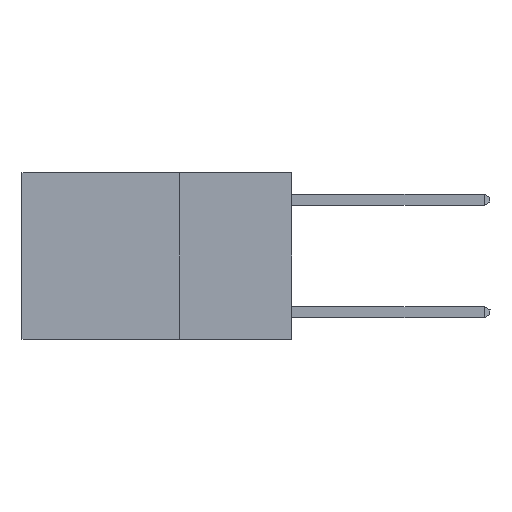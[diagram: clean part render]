
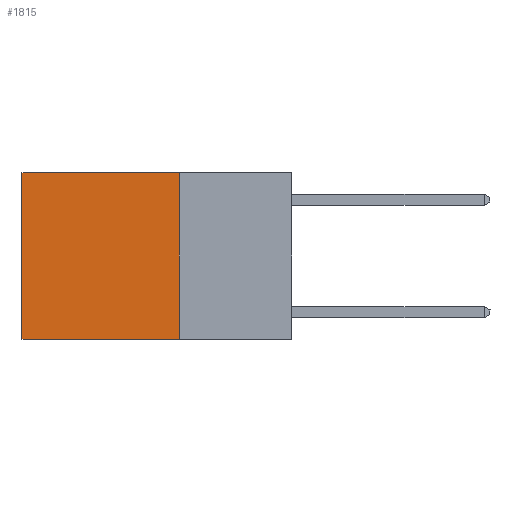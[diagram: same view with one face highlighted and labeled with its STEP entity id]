
A CAD part, left-side view. The second image highlights one B-rep face of the part: STEP entity #1815.
In plain terms, the highlighted planar face has unit normal (-1, 0, 0).
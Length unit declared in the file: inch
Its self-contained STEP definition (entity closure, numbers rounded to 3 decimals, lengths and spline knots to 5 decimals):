
#540 = DIRECTION ( 'NONE',  ( 1., 0., 0. ) ) ;
#552 = DIRECTION ( 'NONE',  ( 0., 0., -1. ) ) ;
#561 = EDGE_CURVE ( 'NONE', #2086, #7018, #8521, .T. ) ;
#582 = PLANE ( 'NONE',  #5282 ) ;
#895 = CARTESIAN_POINT ( 'NONE',  ( 0.2625, 0.25, 0. ) ) ;
#999 = VECTOR ( 'NONE', #6874, 39.37008 ) ;
#1040 = VERTEX_POINT ( 'NONE', #4192 ) ;
#1116 = ORIENTED_EDGE ( 'NONE', *, *, #561, .F. ) ;
#1815 = ADVANCED_FACE ( 'NONE', ( #5709 ), #582, .F. ) ;
#2086 = VERTEX_POINT ( 'NONE', #7889 ) ;
#2486 = ORIENTED_EDGE ( 'NONE', *, *, #6714, .F. ) ;
#2563 = CARTESIAN_POINT ( 'NONE',  ( 0.2625, 0.25, 0. ) ) ;
#2573 = DIRECTION ( 'NONE',  ( 0., 1., 0. ) ) ;
#2875 = CARTESIAN_POINT ( 'NONE',  ( 0.2625, 0.6, 0. ) ) ;
#3490 = LINE ( 'NONE', #6027, #999 ) ;
#3735 = ORIENTED_EDGE ( 'NONE', *, *, #10109, .T. ) ;
#3865 = EDGE_LOOP ( 'NONE', ( #3735, #1116, #2486, #6173 ) ) ;
#4192 = CARTESIAN_POINT ( 'NONE',  ( 0.2625, 0.6, 0. ) ) ;
#4389 = LINE ( 'NONE', #9360, #6615 ) ;
#4550 = DIRECTION ( 'NONE',  ( 0., 0., -1. ) ) ;
#5282 = AXIS2_PLACEMENT_3D ( 'NONE', #895, #540, #552 ) ;
#5709 = FACE_OUTER_BOUND ( 'NONE', #3865, .T. ) ;
#6027 = CARTESIAN_POINT ( 'NONE',  ( 0.2625, 0.25, 0. ) ) ;
#6079 = VERTEX_POINT ( 'NONE', #2563 ) ;
#6173 = ORIENTED_EDGE ( 'NONE', *, *, #7331, .T. ) ;
#6615 = VECTOR ( 'NONE', #6859, 39.37008 ) ;
#6714 = EDGE_CURVE ( 'NONE', #6079, #2086, #3490, .T. ) ;
#6859 = DIRECTION ( 'NONE',  ( 0., 1., 0. ) ) ;
#6874 = DIRECTION ( 'NONE',  ( 0., 0., -1. ) ) ;
#6929 = CARTESIAN_POINT ( 'NONE',  ( 0.2625, 0.25, -0.37 ) ) ;
#7018 = VERTEX_POINT ( 'NONE', #9790 ) ;
#7331 = EDGE_CURVE ( 'NONE', #6079, #1040, #4389, .T. ) ;
#7889 = CARTESIAN_POINT ( 'NONE',  ( 0.2625, 0.25, -0.37 ) ) ;
#8263 = VECTOR ( 'NONE', #2573, 39.37008 ) ;
#8452 = VECTOR ( 'NONE', #4550, 39.37008 ) ;
#8521 = LINE ( 'NONE', #6929, #8263 ) ;
#9360 = CARTESIAN_POINT ( 'NONE',  ( 0.2625, 0.25, 0. ) ) ;
#9790 = CARTESIAN_POINT ( 'NONE',  ( 0.2625, 0.6, -0.37 ) ) ;
#10109 = EDGE_CURVE ( 'NONE', #1040, #7018, #10644, .T. ) ;
#10644 = LINE ( 'NONE', #2875, #8452 ) ;
